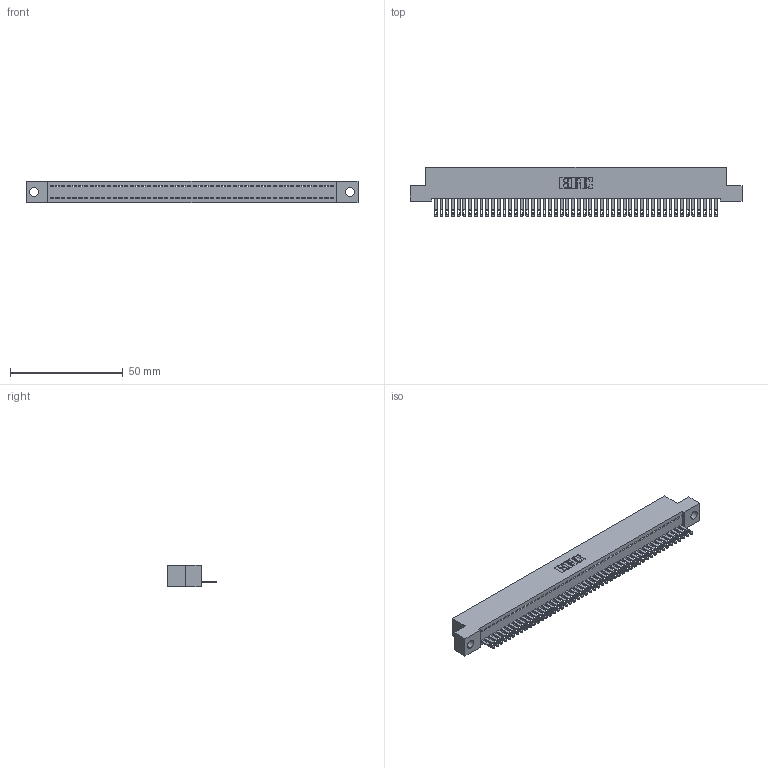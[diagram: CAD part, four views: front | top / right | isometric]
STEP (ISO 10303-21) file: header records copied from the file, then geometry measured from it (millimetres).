
FILE_DESCRIPTION (( 'STEP AP203' ), '1' );
FILE_NAME ('892-050-500-104.STEP', '2020-09-21T17:46:26', ( '' ), ( '' ), 'SwSTEP 2.0', 'SolidWorks 2020', '' );
FILE_SCHEMA (( 'CONFIG_CONTROL_DESIGN' ));
Length unit declared in the file: inch
Products named in the file (3): 842 Part_.156 TH; 345-292-001_345-293-100; 892-050-500-104
Assembly tree (51 placements, depth 2):
  892-050-500-104
    842 Part_.156 TH
    345-292-001_345-293-100  x50
Bounding box: 147.32 x 21.85 x 9.4 mm (x, y, z)
Volume: 12890.4 mm3; surface area: 18995.6 mm2
Topology: 51 solids, 51 shells, 2810 faces, 8699 edges, 5798 vertices
Faces by surface type: plane 1866, cylinder 944
Entity records: 29333 total; most frequent: CARTESIAN_POINT 5064, ORIENTED_EDGE 5050, DIRECTION 4257, EDGE_CURVE 2525, VECTOR 2393, LINE 2393, VERTEX_POINT 1682, AXIS2_PLACEMENT_3D 932
